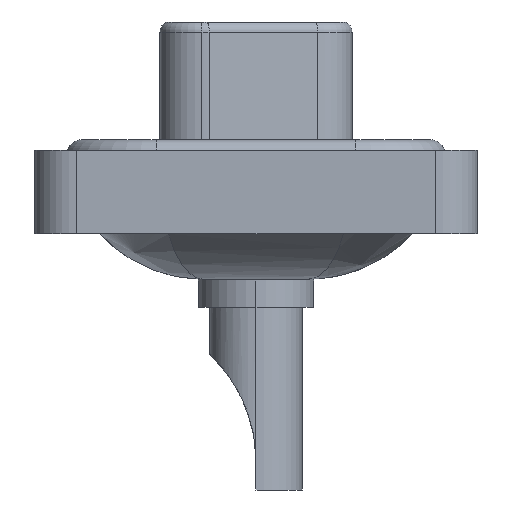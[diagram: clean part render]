
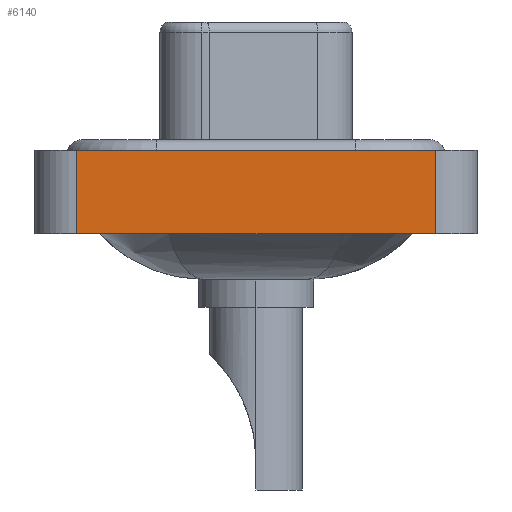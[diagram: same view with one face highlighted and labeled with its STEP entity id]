
A CAD part, left-side view. The second image highlights one B-rep face of the part: STEP entity #6140.
In plain terms, the highlighted planar face has unit normal (-1, 0, 0).
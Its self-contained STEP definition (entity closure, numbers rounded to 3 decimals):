
#336 = EDGE_CURVE ( 'NONE', #6115, #9720, #12019, .T. ) ;
#500 = CARTESIAN_POINT ( 'NONE',  ( -7.3, -8.55, 0.4 ) ) ;
#992 = DIRECTION ( 'NONE',  ( 0., 0., 1. ) ) ;
#2239 = LINE ( 'NONE', #12327, #16354 ) ;
#2337 = AXIS2_PLACEMENT_3D ( 'NONE', #5233, #2689, #11514 ) ;
#2689 = DIRECTION ( 'NONE',  ( -1., 0., 0. ) ) ;
#2729 = VERTEX_POINT ( 'NONE', #10592 ) ;
#3366 = ORIENTED_EDGE ( 'NONE', *, *, #8751, .T. ) ;
#3961 = CARTESIAN_POINT ( 'NONE',  ( -7.3, 8.55, 0.4 ) ) ;
#4827 = CARTESIAN_POINT ( 'NONE',  ( -7.3, -8.55, 0.4 ) ) ;
#4920 = DIRECTION ( 'NONE',  ( 0., 0., 1. ) ) ;
#5233 = CARTESIAN_POINT ( 'NONE',  ( -7.3, -8.55, -3.6 ) ) ;
#5912 = EDGE_LOOP ( 'NONE', ( #13136, #15249, #16052, #3366 ) ) ;
#6115 = VERTEX_POINT ( 'NONE', #3961 ) ;
#6140 = ADVANCED_FACE ( 'NONE', ( #11602 ), #7836, .T. ) ;
#7488 = CARTESIAN_POINT ( 'NONE',  ( -7.3, -8.55, -3.6 ) ) ;
#7836 = PLANE ( 'NONE',  #2337 ) ;
#8249 = DIRECTION ( 'NONE',  ( 0., -1., 0. ) ) ;
#8751 = EDGE_CURVE ( 'NONE', #2729, #10943, #2239, .T. ) ;
#9225 = VECTOR ( 'NONE', #992, 1000. ) ;
#9720 = VERTEX_POINT ( 'NONE', #4827 ) ;
#10042 = CARTESIAN_POINT ( 'NONE',  ( -7.3, 8.55, -3.6 ) ) ;
#10167 = LINE ( 'NONE', #7488, #9225 ) ;
#10176 = VECTOR ( 'NONE', #8249, 1000. ) ;
#10204 = LINE ( 'NONE', #10042, #15970 ) ;
#10592 = CARTESIAN_POINT ( 'NONE',  ( -7.3, 8.55, -3.6 ) ) ;
#10943 = VERTEX_POINT ( 'NONE', #16325 ) ;
#11315 = DIRECTION ( 'NONE',  ( 0., -1., 0. ) ) ;
#11514 = DIRECTION ( 'NONE',  ( 0., 0., 1. ) ) ;
#11602 = FACE_OUTER_BOUND ( 'NONE', #5912, .T. ) ;
#12019 = LINE ( 'NONE', #500, #10176 ) ;
#12327 = CARTESIAN_POINT ( 'NONE',  ( -7.3, -8.55, -3.6 ) ) ;
#12714 = EDGE_CURVE ( 'NONE', #2729, #6115, #10204, .T. ) ;
#13136 = ORIENTED_EDGE ( 'NONE', *, *, #16081, .T. ) ;
#15249 = ORIENTED_EDGE ( 'NONE', *, *, #336, .F. ) ;
#15970 = VECTOR ( 'NONE', #4920, 1000. ) ;
#16052 = ORIENTED_EDGE ( 'NONE', *, *, #12714, .F. ) ;
#16081 = EDGE_CURVE ( 'NONE', #10943, #9720, #10167, .T. ) ;
#16325 = CARTESIAN_POINT ( 'NONE',  ( -7.3, -8.55, -3.6 ) ) ;
#16354 = VECTOR ( 'NONE', #11315, 1000. ) ;
